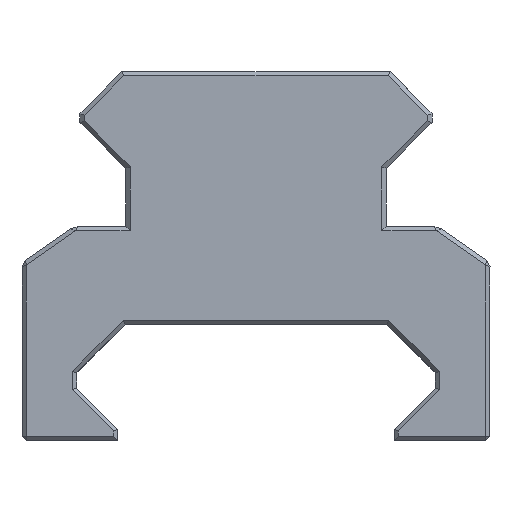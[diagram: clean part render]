
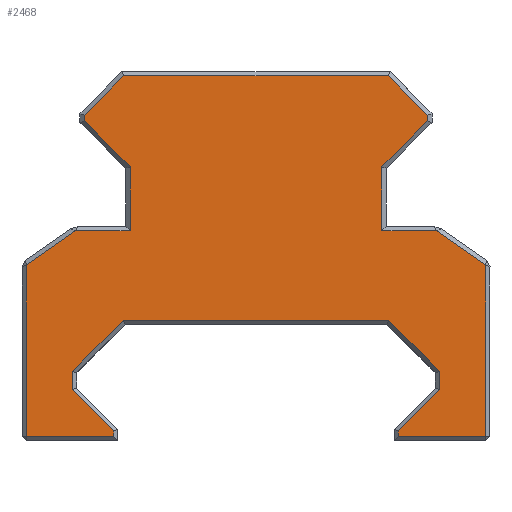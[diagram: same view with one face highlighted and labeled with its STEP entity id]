
A CAD part, front view. The second image highlights one B-rep face of the part: STEP entity #2468.
In plain terms, the highlighted planar face has unit normal (0, -1, 0).
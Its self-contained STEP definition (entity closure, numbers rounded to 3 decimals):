
#140=FACE_OUTER_BOUND('',#284,.T.);
#284=EDGE_LOOP('',(#2032,#2033,#2034,#2035,#2036,#2037,#2038,#2039,#2040,
#2041,#2042,#2043,#2044,#2045,#2046,#2047,#2048,#2049,#2050,#2051,#2052,
#2053,#2054,#2055,#2056,#2057));
#377=LINE('',#3458,#709);
#385=LINE('',#3476,#717);
#391=LINE('',#3488,#723);
#397=LINE('',#3500,#729);
#403=LINE('',#3512,#735);
#409=LINE('',#3523,#741);
#414=LINE('',#3533,#746);
#419=LINE('',#3543,#751);
#424=LINE('',#3553,#756);
#429=LINE('',#3563,#761);
#441=LINE('',#3588,#773);
#452=LINE('',#3611,#784);
#461=LINE('',#3631,#793);
#466=LINE('',#3638,#798);
#474=LINE('',#3652,#806);
#481=LINE('',#3663,#813);
#486=LINE('',#3673,#818);
#492=LINE('',#3685,#824);
#498=LINE('',#3697,#830);
#504=LINE('',#3709,#836);
#510=LINE('',#3721,#842);
#516=LINE('',#3733,#848);
#522=LINE('',#3745,#854);
#527=LINE('',#3754,#859);
#533=LINE('',#3764,#865);
#542=LINE('',#3779,#874);
#709=VECTOR('',#2795,10.);
#717=VECTOR('',#2809,10.);
#723=VECTOR('',#2819,10.);
#729=VECTOR('',#2829,10.);
#735=VECTOR('',#2839,10.);
#741=VECTOR('',#2849,10.);
#746=VECTOR('',#2858,10.);
#751=VECTOR('',#2867,10.);
#756=VECTOR('',#2876,10.);
#761=VECTOR('',#2885,10.);
#773=VECTOR('',#2905,10.);
#784=VECTOR('',#2924,10.);
#793=VECTOR('',#2939,10.);
#798=VECTOR('',#2948,10.);
#806=VECTOR('',#2964,10.);
#813=VECTOR('',#2977,10.);
#818=VECTOR('',#2986,10.);
#824=VECTOR('',#2996,10.);
#830=VECTOR('',#3006,10.);
#836=VECTOR('',#3016,10.);
#842=VECTOR('',#3026,10.);
#848=VECTOR('',#3036,10.);
#854=VECTOR('',#3046,10.);
#859=VECTOR('',#3055,10.);
#865=VECTOR('',#3065,10.);
#874=VECTOR('',#3082,10.);
#1031=VERTEX_POINT('',#3437);
#1037=VERTEX_POINT('',#3451);
#1039=VERTEX_POINT('',#3457);
#1045=VERTEX_POINT('',#3471);
#1046=VERTEX_POINT('',#3475);
#1050=VERTEX_POINT('',#3487);
#1054=VERTEX_POINT('',#3499);
#1058=VERTEX_POINT('',#3511);
#1061=VERTEX_POINT('',#3522);
#1064=VERTEX_POINT('',#3532);
#1067=VERTEX_POINT('',#3542);
#1070=VERTEX_POINT('',#3552);
#1073=VERTEX_POINT('',#3562);
#1082=VERTEX_POINT('',#3584);
#1090=VERTEX_POINT('',#3607);
#1094=VERTEX_POINT('',#3621);
#1098=VERTEX_POINT('',#3630);
#1100=VERTEX_POINT('',#3651);
#1101=VERTEX_POINT('',#3662);
#1104=VERTEX_POINT('',#3672);
#1108=VERTEX_POINT('',#3684);
#1112=VERTEX_POINT('',#3696);
#1116=VERTEX_POINT('',#3708);
#1120=VERTEX_POINT('',#3720);
#1124=VERTEX_POINT('',#3732);
#1128=VERTEX_POINT('',#3744);
#1257=EDGE_CURVE('',#1031,#1039,#377,.T.);
#1265=EDGE_CURVE('',#1039,#1046,#385,.T.);
#1271=EDGE_CURVE('',#1046,#1050,#391,.T.);
#1277=EDGE_CURVE('',#1050,#1054,#397,.T.);
#1283=EDGE_CURVE('',#1054,#1058,#403,.T.);
#1289=EDGE_CURVE('',#1058,#1061,#409,.T.);
#1294=EDGE_CURVE('',#1061,#1064,#414,.T.);
#1299=EDGE_CURVE('',#1064,#1067,#419,.T.);
#1304=EDGE_CURVE('',#1067,#1070,#424,.T.);
#1309=EDGE_CURVE('',#1070,#1073,#429,.T.);
#1321=EDGE_CURVE('',#1073,#1082,#441,.T.);
#1332=EDGE_CURVE('',#1082,#1090,#452,.T.);
#1341=EDGE_CURVE('',#1094,#1098,#461,.T.);
#1346=EDGE_CURVE('',#1090,#1094,#466,.T.);
#1354=EDGE_CURVE('',#1098,#1100,#474,.T.);
#1361=EDGE_CURVE('',#1100,#1101,#481,.T.);
#1366=EDGE_CURVE('',#1101,#1104,#486,.T.);
#1372=EDGE_CURVE('',#1104,#1108,#492,.T.);
#1378=EDGE_CURVE('',#1108,#1112,#498,.T.);
#1384=EDGE_CURVE('',#1112,#1116,#504,.T.);
#1390=EDGE_CURVE('',#1116,#1120,#510,.T.);
#1396=EDGE_CURVE('',#1120,#1124,#516,.T.);
#1402=EDGE_CURVE('',#1124,#1128,#522,.T.);
#1407=EDGE_CURVE('',#1128,#1045,#527,.T.);
#1413=EDGE_CURVE('',#1045,#1037,#533,.T.);
#1422=EDGE_CURVE('',#1037,#1031,#542,.T.);
#2032=ORIENTED_EDGE('',*,*,#1341,.F.);
#2033=ORIENTED_EDGE('',*,*,#1346,.F.);
#2034=ORIENTED_EDGE('',*,*,#1332,.F.);
#2035=ORIENTED_EDGE('',*,*,#1321,.F.);
#2036=ORIENTED_EDGE('',*,*,#1309,.F.);
#2037=ORIENTED_EDGE('',*,*,#1304,.F.);
#2038=ORIENTED_EDGE('',*,*,#1299,.F.);
#2039=ORIENTED_EDGE('',*,*,#1294,.F.);
#2040=ORIENTED_EDGE('',*,*,#1289,.F.);
#2041=ORIENTED_EDGE('',*,*,#1283,.F.);
#2042=ORIENTED_EDGE('',*,*,#1277,.F.);
#2043=ORIENTED_EDGE('',*,*,#1271,.F.);
#2044=ORIENTED_EDGE('',*,*,#1265,.F.);
#2045=ORIENTED_EDGE('',*,*,#1257,.F.);
#2046=ORIENTED_EDGE('',*,*,#1422,.F.);
#2047=ORIENTED_EDGE('',*,*,#1413,.F.);
#2048=ORIENTED_EDGE('',*,*,#1407,.F.);
#2049=ORIENTED_EDGE('',*,*,#1402,.F.);
#2050=ORIENTED_EDGE('',*,*,#1396,.F.);
#2051=ORIENTED_EDGE('',*,*,#1390,.F.);
#2052=ORIENTED_EDGE('',*,*,#1384,.F.);
#2053=ORIENTED_EDGE('',*,*,#1378,.F.);
#2054=ORIENTED_EDGE('',*,*,#1372,.F.);
#2055=ORIENTED_EDGE('',*,*,#1366,.F.);
#2056=ORIENTED_EDGE('',*,*,#1361,.F.);
#2057=ORIENTED_EDGE('',*,*,#1354,.F.);
#2326=PLANE('',#2636);
#2468=ADVANCED_FACE('',(#140),#2326,.F.);
#2636=AXIS2_PLACEMENT_3D('',#3910,#3200,#3201);
#2795=DIRECTION('',(1.,0.,0.));
#2809=DIRECTION('',(0.,0.,1.));
#2819=DIRECTION('',(-0.707,0.,0.707));
#2829=DIRECTION('',(0.,0.,1.));
#2839=DIRECTION('',(0.707,0.,0.707));
#2849=DIRECTION('',(1.,0.,0.));
#2858=DIRECTION('',(0.707,0.,-0.707));
#2867=DIRECTION('',(0.,0.,-1.));
#2876=DIRECTION('',(-0.707,0.,-0.707));
#2885=DIRECTION('',(0.,0.,-1.));
#2905=DIRECTION('',(1.,0.,0.));
#2924=DIRECTION('',(0.819,0.,-0.574));
#2939=DIRECTION('',(-1.,0.,0.));
#2948=DIRECTION('',(0.,0.,-1.));
#2964=DIRECTION('',(0.,0.,1.));
#2977=DIRECTION('',(0.707,0.,0.707));
#2986=DIRECTION('',(0.,0.,1.));
#2996=DIRECTION('',(-0.707,0.,0.707));
#3006=DIRECTION('',(-1.,0.,0.));
#3016=DIRECTION('',(-0.707,0.,-0.707));
#3026=DIRECTION('',(0.,0.,-1.));
#3036=DIRECTION('',(0.707,0.,-0.707));
#3046=DIRECTION('',(0.,0.,-1.));
#3055=DIRECTION('',(-1.,0.,0.));
#3065=DIRECTION('',(0.,0.,1.));
#3082=DIRECTION('',(0.819,0.,0.574));
#3200=DIRECTION('center_axis',(0.,1.,0.));
#3201=DIRECTION('ref_axis',(1.,0.,0.));
#3437=CARTESIAN_POINT('',(-10.886,0.,-6.782));
#3451=CARTESIAN_POINT('',(-13.843,0.,-8.852));
#3457=CARTESIAN_POINT('',(-7.582,0.,-6.782));
#3458=CARTESIAN_POINT('',(-5.483,0.,-6.782));
#3471=CARTESIAN_POINT('',(-13.843,0.,-19.164));
#3475=CARTESIAN_POINT('',(-7.582,0.,-2.93));
#3476=CARTESIAN_POINT('',(-7.582,0.,-7.42));
#3487=CARTESIAN_POINT('',(-10.35,0.,-0.161));
#3488=CARTESIAN_POINT('',(-4.378,0.,-6.134));
#3499=CARTESIAN_POINT('',(-10.35,0.,0.161));
#3500=CARTESIAN_POINT('',(-10.35,0.,-4.289));
#3511=CARTESIAN_POINT('',(-7.972,0.,2.54));
#3512=CARTESIAN_POINT('',(-9.918,0.,0.594));
#3522=CARTESIAN_POINT('',(7.972,0.,2.54));
#3523=CARTESIAN_POINT('',(-4.039,0.,2.54));
#3532=CARTESIAN_POINT('',(10.35,0.,0.161));
#3533=CARTESIAN_POINT('',(8.655,0.,1.857));
#3542=CARTESIAN_POINT('',(10.35,0.,-0.161));
#3543=CARTESIAN_POINT('',(10.35,0.,-4.023));
#3552=CARTESIAN_POINT('',(7.582,0.,-2.93));
#3553=CARTESIAN_POINT('',(5.762,0.,-4.75));
#3562=CARTESIAN_POINT('',(7.582,0.,-6.782));
#3563=CARTESIAN_POINT('',(7.582,0.,-5.674));
#3584=CARTESIAN_POINT('',(10.886,0.,-6.782));
#3588=CARTESIAN_POINT('',(3.918,0.,-6.782));
#3607=CARTESIAN_POINT('',(13.843,0.,-8.852));
#3611=CARTESIAN_POINT('',(7.561,0.,-4.453));
#3621=CARTESIAN_POINT('',(13.843,0.,-19.164));
#3630=CARTESIAN_POINT('',(8.572,0.,-19.164));
#3631=CARTESIAN_POINT('',(7.048,0.,-19.164));
#3638=CARTESIAN_POINT('',(13.843,0.,-8.516));
#3651=CARTESIAN_POINT('',(8.572,0.,-18.85));
#3652=CARTESIAN_POINT('',(8.572,0.,-13.865));
#3662=CARTESIAN_POINT('',(11.049,0.,-16.374));
#3663=CARTESIAN_POINT('',(9.027,0.,-18.396));
#3672=CARTESIAN_POINT('',(11.049,0.,-15.249));
#3673=CARTESIAN_POINT('',(11.049,0.,-12.29));
#3684=CARTESIAN_POINT('',(7.992,0.,-12.192));
#3685=CARTESIAN_POINT('',(6.515,0.,-10.715));
#3696=CARTESIAN_POINT('',(-7.992,0.,-12.192));
#3697=CARTESIAN_POINT('',(3.943,0.,-12.192));
#3708=CARTESIAN_POINT('',(-11.049,0.,-15.249));
#3709=CARTESIAN_POINT('',(-5.061,0.,-9.261));
#3720=CARTESIAN_POINT('',(-11.049,0.,-16.374));
#3721=CARTESIAN_POINT('',(-11.049,0.,-11.833));
#3732=CARTESIAN_POINT('',(-8.572,0.,-18.85));
#3733=CARTESIAN_POINT('',(-10.265,0.,-17.158));
#3744=CARTESIAN_POINT('',(-8.572,0.,-19.164));
#3745=CARTESIAN_POINT('',(-8.572,0.,-13.529));
#3754=CARTESIAN_POINT('',(-4.159,0.,-19.164));
#3764=CARTESIAN_POINT('',(-13.843,0.,-13.865));
#3779=CARTESIAN_POINT('',(-9.126,0.,-5.549));
#3910=CARTESIAN_POINT('Origin',(0.,0.,-8.312));
